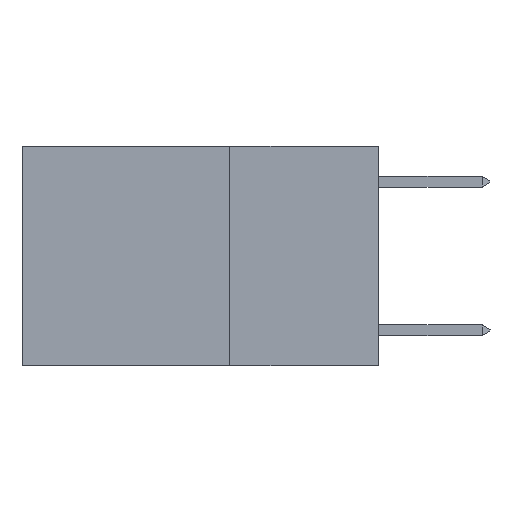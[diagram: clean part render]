
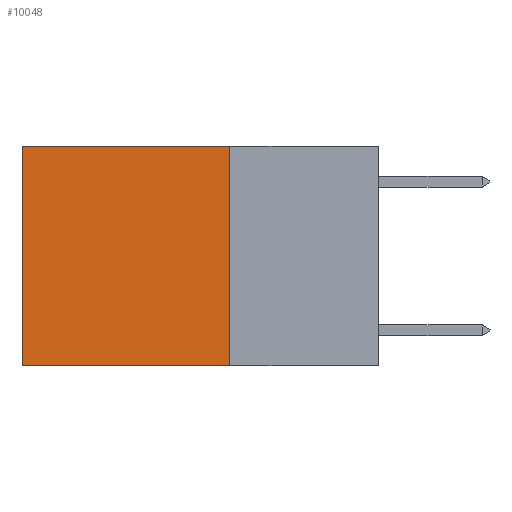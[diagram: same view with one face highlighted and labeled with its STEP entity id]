
A CAD part, left-side view. The second image highlights one B-rep face of the part: STEP entity #10048.
In plain terms, the highlighted planar face has unit normal (-1, 0, 0).
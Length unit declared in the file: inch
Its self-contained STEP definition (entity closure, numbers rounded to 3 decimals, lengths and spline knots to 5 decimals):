
#562 = CARTESIAN_POINT ( 'NONE',  ( 0.2625, 0.6, 0. ) ) ;
#751 = VECTOR ( 'NONE', #11675, 39.37008 ) ;
#1148 = CARTESIAN_POINT ( 'NONE',  ( 0.2625, 0.25, 0. ) ) ;
#1622 = CARTESIAN_POINT ( 'NONE',  ( 0.2625, 0.25, 0. ) ) ;
#2068 = AXIS2_PLACEMENT_3D ( 'NONE', #8900, #13394, #4652 ) ;
#2144 = EDGE_CURVE ( 'NONE', #13889, #15250, #13307, .T. ) ;
#3329 = ORIENTED_EDGE ( 'NONE', *, *, #6521, .F. ) ;
#3871 = LINE ( 'NONE', #15527, #9809 ) ;
#4135 = LINE ( 'NONE', #4776, #14786 ) ;
#4652 = DIRECTION ( 'NONE',  ( 0., 0., -1. ) ) ;
#4714 = PLANE ( 'NONE',  #2068 ) ;
#4776 = CARTESIAN_POINT ( 'NONE',  ( 0.2625, 0.25, 0. ) ) ;
#5624 = EDGE_CURVE ( 'NONE', #17671, #15250, #3871, .T. ) ;
#6437 = VECTOR ( 'NONE', #10556, 39.37008 ) ;
#6521 = EDGE_CURVE ( 'NONE', #14189, #13889, #15606, .T. ) ;
#7442 = DIRECTION ( 'NONE',  ( 0., 1., 0. ) ) ;
#8900 = CARTESIAN_POINT ( 'NONE',  ( 0.2625, 0.25, 0. ) ) ;
#9013 = ORIENTED_EDGE ( 'NONE', *, *, #10094, .T. ) ;
#9181 = CARTESIAN_POINT ( 'NONE',  ( 0.2625, 0.25, -0.37 ) ) ;
#9809 = VECTOR ( 'NONE', #16845, 39.37008 ) ;
#10048 = ADVANCED_FACE ( 'NONE', ( #13693 ), #4714, .F. ) ;
#10094 = EDGE_CURVE ( 'NONE', #14189, #17671, #4135, .T. ) ;
#10556 = DIRECTION ( 'NONE',  ( 0., 1., 0. ) ) ;
#11191 = ORIENTED_EDGE ( 'NONE', *, *, #2144, .F. ) ;
#11675 = DIRECTION ( 'NONE',  ( 0., 0., -1. ) ) ;
#13307 = LINE ( 'NONE', #16431, #6437 ) ;
#13394 = DIRECTION ( 'NONE',  ( 1., 0., 0. ) ) ;
#13603 = CARTESIAN_POINT ( 'NONE',  ( 0.2625, 0.6, -0.37 ) ) ;
#13693 = FACE_OUTER_BOUND ( 'NONE', #16788, .T. ) ;
#13889 = VERTEX_POINT ( 'NONE', #9181 ) ;
#14189 = VERTEX_POINT ( 'NONE', #1148 ) ;
#14786 = VECTOR ( 'NONE', #7442, 39.37008 ) ;
#15250 = VERTEX_POINT ( 'NONE', #13603 ) ;
#15527 = CARTESIAN_POINT ( 'NONE',  ( 0.2625, 0.6, 0. ) ) ;
#15606 = LINE ( 'NONE', #1622, #751 ) ;
#16431 = CARTESIAN_POINT ( 'NONE',  ( 0.2625, 0.25, -0.37 ) ) ;
#16788 = EDGE_LOOP ( 'NONE', ( #17997, #11191, #3329, #9013 ) ) ;
#16845 = DIRECTION ( 'NONE',  ( 0., 0., -1. ) ) ;
#17671 = VERTEX_POINT ( 'NONE', #562 ) ;
#17997 = ORIENTED_EDGE ( 'NONE', *, *, #5624, .T. ) ;
